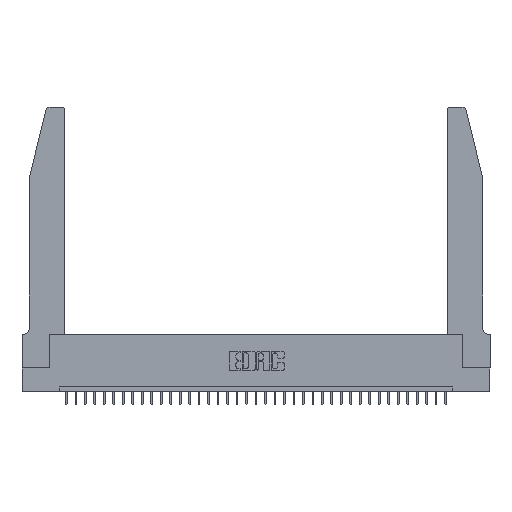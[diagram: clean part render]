
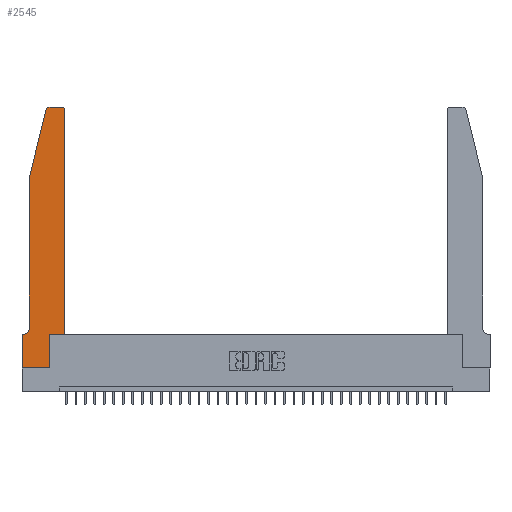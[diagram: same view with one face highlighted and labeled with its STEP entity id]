
A CAD part, top view. The second image highlights one B-rep face of the part: STEP entity #2545.
In plain terms, the highlighted planar face has unit normal (0, 0, 1).
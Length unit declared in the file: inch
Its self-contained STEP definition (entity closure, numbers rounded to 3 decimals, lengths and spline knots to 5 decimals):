
#35 = VERTEX_POINT ( 'NONE', #26270 ) ;
#953 = VECTOR ( 'NONE', #5681, 39.37008 ) ;
#1241 = VECTOR ( 'NONE', #27740, 39.37008 ) ;
#1319 = CARTESIAN_POINT ( 'NONE',  ( 0.0055, 0.35, 0.37 ) ) ;
#1485 = EDGE_CURVE ( 'NONE', #28636, #25341, #17246, .T. ) ;
#1737 = DIRECTION ( 'NONE',  ( 1., 0., 0. ) ) ;
#2151 = DIRECTION ( 'NONE',  ( 0., 0., 1. ) ) ;
#2545 = ADVANCED_FACE ( 'NONE', ( #18882 ), #10347, .T. ) ;
#2737 = LINE ( 'NONE', #13654, #25545 ) ;
#2861 = LINE ( 'NONE', #5592, #7314 ) ;
#3174 = CARTESIAN_POINT ( 'NONE',  ( 0.2605, 2.75, 0.37 ) ) ;
#3867 = ORIENTED_EDGE ( 'NONE', *, *, #14602, .T. ) ;
#4080 = LINE ( 'NONE', #31811, #19442 ) ;
#4879 = DIRECTION ( 'NONE',  ( 1., 0., 0. ) ) ;
#5252 = DIRECTION ( 'NONE',  ( 1., 0., 0. ) ) ;
#5592 = CARTESIAN_POINT ( 'NONE',  ( 0.0755, 2., 0.37 ) ) ;
#5595 = VECTOR ( 'NONE', #13920, 39.37008 ) ;
#5633 = LINE ( 'NONE', #16725, #1241 ) ;
#5681 = DIRECTION ( 'NONE',  ( -1., 0., 0. ) ) ;
#5771 = ORIENTED_EDGE ( 'NONE', *, *, #13413, .T. ) ;
#5857 = CARTESIAN_POINT ( 'NONE',  ( 0.0755, 0.35, 0.37 ) ) ;
#7314 = VECTOR ( 'NONE', #11416, 39.37008 ) ;
#8410 = CARTESIAN_POINT ( 'NONE',  ( 0., 0., 0.37 ) ) ;
#8726 = EDGE_CURVE ( 'NONE', #35, #19259, #16519, .T. ) ;
#8852 = AXIS2_PLACEMENT_3D ( 'NONE', #13281, #21979, #27556 ) ;
#9305 = CARTESIAN_POINT ( 'NONE',  ( 0., 0.35, 0.37 ) ) ;
#9691 = VECTOR ( 'NONE', #11059, 39.37008 ) ;
#10347 = PLANE ( 'NONE',  #26950 ) ;
#10607 = EDGE_CURVE ( 'NONE', #17062, #10666, #30499, .T. ) ;
#10666 = VERTEX_POINT ( 'NONE', #9305 ) ;
#10757 = CARTESIAN_POINT ( 'NONE',  ( 0.0755, 0.42, 0.37 ) ) ;
#11059 = DIRECTION ( 'NONE',  ( 0., 1., 0. ) ) ;
#11416 = DIRECTION ( 'NONE',  ( -0.239, -0.971, 0. ) ) ;
#11976 = CARTESIAN_POINT ( 'NONE',  ( 0.2865, 0.35, 0.37 ) ) ;
#12094 = CARTESIAN_POINT ( 'NONE',  ( 0.4505, 2.72, 0.37 ) ) ;
#12194 = EDGE_CURVE ( 'NONE', #25341, #35, #2737, .T. ) ;
#12314 = AXIS2_PLACEMENT_3D ( 'NONE', #18709, #21793, #5252 ) ;
#13035 = EDGE_CURVE ( 'NONE', #10666, #19592, #5633, .T. ) ;
#13182 = EDGE_CURVE ( 'NONE', #19592, #28636, #17092, .T. ) ;
#13281 = CARTESIAN_POINT ( 'NONE',  ( 0.0055, 0.42, 0.37 ) ) ;
#13413 = EDGE_CURVE ( 'NONE', #26794, #27506, #23299, .T. ) ;
#13437 = CARTESIAN_POINT ( 'NONE',  ( 0., 0.35, 0.37 ) ) ;
#13654 = CARTESIAN_POINT ( 'NONE',  ( 0.4505, 0.35, 0.37 ) ) ;
#13754 = CARTESIAN_POINT ( 'NONE',  ( 0.2865, 0.35, 0.37 ) ) ;
#13920 = DIRECTION ( 'NONE',  ( -1., 0., 0. ) ) ;
#14391 = DIRECTION ( 'NONE',  ( 1., 0., 0. ) ) ;
#14519 = ORIENTED_EDGE ( 'NONE', *, *, #8726, .T. ) ;
#14602 = EDGE_CURVE ( 'NONE', #35525, #17062, #27359, .T. ) ;
#15324 = ORIENTED_EDGE ( 'NONE', *, *, #33600, .T. ) ;
#16280 = DIRECTION ( 'NONE',  ( 0., 0., 1. ) ) ;
#16519 = LINE ( 'NONE', #17784, #9691 ) ;
#16725 = CARTESIAN_POINT ( 'NONE',  ( 0., 0., 0.37 ) ) ;
#17062 = VERTEX_POINT ( 'NONE', #1319 ) ;
#17092 = LINE ( 'NONE', #28117, #17520 ) ;
#17100 = CARTESIAN_POINT ( 'NONE',  ( 0.25487, 2.72718, 0.37 ) ) ;
#17246 = LINE ( 'NONE', #11976, #26339 ) ;
#17520 = VECTOR ( 'NONE', #14391, 39.37008 ) ;
#17784 = CARTESIAN_POINT ( 'NONE',  ( 0.4505, 0.35, 0.37 ) ) ;
#17910 = CARTESIAN_POINT ( 'NONE',  ( 0.0755, 2., 0.37 ) ) ;
#18080 = DIRECTION ( 'NONE',  ( 0., -1., 0. ) ) ;
#18471 = CARTESIAN_POINT ( 'NONE',  ( 0.4205, 2.72, 0.37 ) ) ;
#18682 = ORIENTED_EDGE ( 'NONE', *, *, #19933, .T. ) ;
#18709 = CARTESIAN_POINT ( 'NONE',  ( 0.284, 2.72, 0.37 ) ) ;
#18882 = FACE_OUTER_BOUND ( 'NONE', #29269, .T. ) ;
#19259 = VERTEX_POINT ( 'NONE', #12094 ) ;
#19442 = VECTOR ( 'NONE', #18080, 39.37008 ) ;
#19592 = VERTEX_POINT ( 'NONE', #8410 ) ;
#19933 = EDGE_CURVE ( 'NONE', #27506, #32326, #2861, .T. ) ;
#20030 = ORIENTED_EDGE ( 'NONE', *, *, #10607, .T. ) ;
#20264 = ORIENTED_EDGE ( 'NONE', *, *, #29541, .T. ) ;
#20425 = EDGE_CURVE ( 'NONE', #21111, #26794, #28020, .T. ) ;
#21111 = VERTEX_POINT ( 'NONE', #21750 ) ;
#21750 = CARTESIAN_POINT ( 'NONE',  ( 0.4205, 2.75, 0.37 ) ) ;
#21793 = DIRECTION ( 'NONE',  ( 0., 0., 1. ) ) ;
#21979 = DIRECTION ( 'NONE',  ( 0., 0., -1. ) ) ;
#22681 = ORIENTED_EDGE ( 'NONE', *, *, #1485, .T. ) ;
#23035 = DIRECTION ( 'NONE',  ( 0., 1., 0. ) ) ;
#23299 = CIRCLE ( 'NONE', #12314, 0.03 ) ;
#24249 = ORIENTED_EDGE ( 'NONE', *, *, #12194, .T. ) ;
#25341 = VERTEX_POINT ( 'NONE', #13754 ) ;
#25545 = VECTOR ( 'NONE', #30459, 39.37008 ) ;
#25561 = AXIS2_PLACEMENT_3D ( 'NONE', #18471, #16280, #1737 ) ;
#26270 = CARTESIAN_POINT ( 'NONE',  ( 0.4505, 0.35, 0.37 ) ) ;
#26339 = VECTOR ( 'NONE', #23035, 39.37008 ) ;
#26794 = VERTEX_POINT ( 'NONE', #30611 ) ;
#26950 = AXIS2_PLACEMENT_3D ( 'NONE', #13437, #2151, #4879 ) ;
#27359 = CIRCLE ( 'NONE', #8852, 0.07 ) ;
#27506 = VERTEX_POINT ( 'NONE', #17100 ) ;
#27556 = DIRECTION ( 'NONE',  ( -1., 0., 0. ) ) ;
#27740 = DIRECTION ( 'NONE',  ( 0., -1., 0. ) ) ;
#28020 = LINE ( 'NONE', #3174, #5595 ) ;
#28117 = CARTESIAN_POINT ( 'NONE',  ( 0., 0., 0.37 ) ) ;
#28636 = VERTEX_POINT ( 'NONE', #30002 ) ;
#29269 = EDGE_LOOP ( 'NONE', ( #35678, #5771, #18682, #15324, #3867, #20030, #33382, #31954, #22681, #24249, #14519, #20264 ) ) ;
#29541 = EDGE_CURVE ( 'NONE', #19259, #21111, #35394, .T. ) ;
#30002 = CARTESIAN_POINT ( 'NONE',  ( 0.2865, 0., 0.37 ) ) ;
#30459 = DIRECTION ( 'NONE',  ( 1., 0., 0. ) ) ;
#30499 = LINE ( 'NONE', #5857, #953 ) ;
#30611 = CARTESIAN_POINT ( 'NONE',  ( 0.284, 2.75, 0.37 ) ) ;
#31811 = CARTESIAN_POINT ( 'NONE',  ( 0.0755, 2., 0.37 ) ) ;
#31954 = ORIENTED_EDGE ( 'NONE', *, *, #13182, .T. ) ;
#32326 = VERTEX_POINT ( 'NONE', #17910 ) ;
#33382 = ORIENTED_EDGE ( 'NONE', *, *, #13035, .T. ) ;
#33600 = EDGE_CURVE ( 'NONE', #32326, #35525, #4080, .T. ) ;
#35394 = CIRCLE ( 'NONE', #25561, 0.03 ) ;
#35525 = VERTEX_POINT ( 'NONE', #10757 ) ;
#35678 = ORIENTED_EDGE ( 'NONE', *, *, #20425, .T. ) ;
